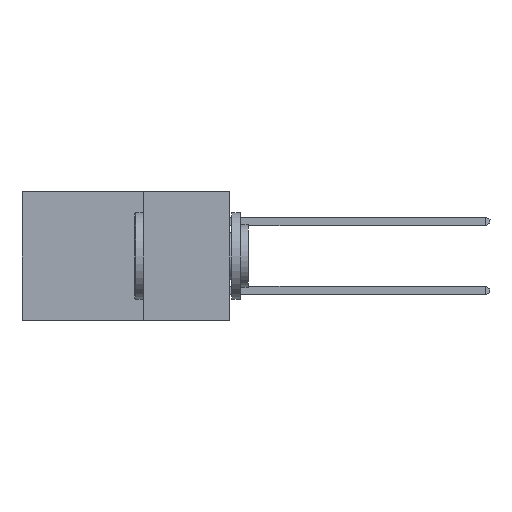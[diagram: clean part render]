
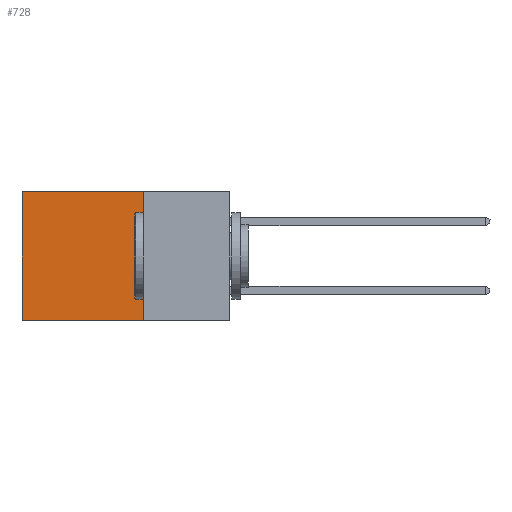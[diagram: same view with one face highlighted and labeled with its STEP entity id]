
A CAD part, left-side view. The second image highlights one B-rep face of the part: STEP entity #728.
In plain terms, the highlighted planar face has unit normal (-1, 0, 0).
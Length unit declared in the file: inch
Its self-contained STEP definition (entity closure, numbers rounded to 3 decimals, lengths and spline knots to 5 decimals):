
#651 = EDGE_CURVE ( 'NONE', #8267, #2548, #8163, .T. ) ;
#728 = ADVANCED_FACE ( 'NONE', ( #2524 ), #1045, .F. ) ;
#758 = VECTOR ( 'NONE', #9007, 39.37008 ) ;
#994 = ORIENTED_EDGE ( 'NONE', *, *, #1457, .F. ) ;
#1045 = PLANE ( 'NONE',  #5294 ) ;
#1276 = VECTOR ( 'NONE', #7137, 39.37008 ) ;
#1376 = LINE ( 'NONE', #5153, #758 ) ;
#1457 = EDGE_CURVE ( 'NONE', #8267, #6220, #7240, .T. ) ;
#1513 = DIRECTION ( 'NONE',  ( 0., 1., 0. ) ) ;
#1811 = DIRECTION ( 'NONE',  ( 0., 0., -1. ) ) ;
#2254 = CARTESIAN_POINT ( 'NONE',  ( 0.2615, 0.25, -0.37 ) ) ;
#2524 = FACE_OUTER_BOUND ( 'NONE', #5996, .T. ) ;
#2548 = VERTEX_POINT ( 'NONE', #3916 ) ;
#2885 = ORIENTED_EDGE ( 'NONE', *, *, #651, .T. ) ;
#3916 = CARTESIAN_POINT ( 'NONE',  ( 0.2615, 0.6, 0. ) ) ;
#4258 = ORIENTED_EDGE ( 'NONE', *, *, #7124, .T. ) ;
#4618 = VECTOR ( 'NONE', #6999, 39.37008 ) ;
#4698 = ORIENTED_EDGE ( 'NONE', *, *, #5955, .F. ) ;
#4781 = CARTESIAN_POINT ( 'NONE',  ( 0.2615, 0.25, -0.37 ) ) ;
#5147 = VECTOR ( 'NONE', #1513, 39.37008 ) ;
#5153 = CARTESIAN_POINT ( 'NONE',  ( 0.2615, 0.6, -0.37 ) ) ;
#5294 = AXIS2_PLACEMENT_3D ( 'NONE', #4781, #7015, #1811 ) ;
#5955 = EDGE_CURVE ( 'NONE', #6220, #7318, #9975, .T. ) ;
#5996 = EDGE_LOOP ( 'NONE', ( #4258, #4698, #994, #2885 ) ) ;
#6215 = CARTESIAN_POINT ( 'NONE',  ( 0.2615, 0.25, -0.37 ) ) ;
#6220 = VERTEX_POINT ( 'NONE', #6215 ) ;
#6999 = DIRECTION ( 'NONE',  ( 0., 1., 0. ) ) ;
#7015 = DIRECTION ( 'NONE',  ( 1., 0., 0. ) ) ;
#7124 = EDGE_CURVE ( 'NONE', #2548, #7318, #1376, .T. ) ;
#7137 = DIRECTION ( 'NONE',  ( 0., 0., -1. ) ) ;
#7240 = LINE ( 'NONE', #8697, #1276 ) ;
#7318 = VERTEX_POINT ( 'NONE', #8109 ) ;
#7925 = CARTESIAN_POINT ( 'NONE',  ( 0.2615, 0.25, 0. ) ) ;
#8109 = CARTESIAN_POINT ( 'NONE',  ( 0.2615, 0.6, -0.37 ) ) ;
#8163 = LINE ( 'NONE', #8465, #5147 ) ;
#8267 = VERTEX_POINT ( 'NONE', #7925 ) ;
#8465 = CARTESIAN_POINT ( 'NONE',  ( 0.2615, 0.25, 0. ) ) ;
#8697 = CARTESIAN_POINT ( 'NONE',  ( 0.2615, 0.25, -0.37 ) ) ;
#9007 = DIRECTION ( 'NONE',  ( 0., 0., -1. ) ) ;
#9975 = LINE ( 'NONE', #2254, #4618 ) ;
